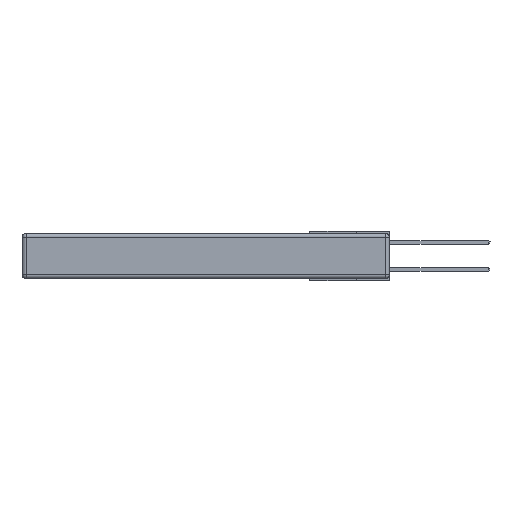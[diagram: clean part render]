
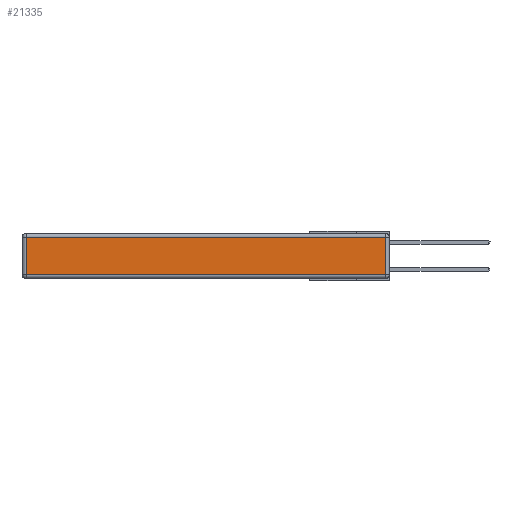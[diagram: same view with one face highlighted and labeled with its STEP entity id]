
A CAD part, left-side view. The second image highlights one B-rep face of the part: STEP entity #21335.
In plain terms, the highlighted planar face has unit normal (-1, 0, 0).
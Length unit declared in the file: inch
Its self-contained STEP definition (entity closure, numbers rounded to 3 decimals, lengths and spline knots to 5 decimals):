
#767 = CARTESIAN_POINT ( 'NONE',  ( 0., 0.03, -0.343 ) ) ;
#1240 = PLANE ( 'NONE',  #9766 ) ;
#1264 = DIRECTION ( 'NONE',  ( 0., 0., -1. ) ) ;
#2374 = CARTESIAN_POINT ( 'NONE',  ( 0., 0.03, -0.03 ) ) ;
#3075 = ORIENTED_EDGE ( 'NONE', *, *, #14206, .T. ) ;
#4648 = ORIENTED_EDGE ( 'NONE', *, *, #5697, .T. ) ;
#4725 = LINE ( 'NONE', #767, #12222 ) ;
#4911 = VECTOR ( 'NONE', #1264, 39.37008 ) ;
#5486 = CARTESIAN_POINT ( 'NONE',  ( 0., 0., -0.313 ) ) ;
#5515 = EDGE_CURVE ( 'NONE', #13794, #26208, #24156, .T. ) ;
#5697 = EDGE_CURVE ( 'NONE', #26208, #15934, #6198, .T. ) ;
#6198 = LINE ( 'NONE', #17628, #4911 ) ;
#6854 = VECTOR ( 'NONE', #22027, 39.37008 ) ;
#7051 = DIRECTION ( 'NONE',  ( 0., 0., 1. ) ) ;
#7062 = ORIENTED_EDGE ( 'NONE', *, *, #5515, .T. ) ;
#7544 = CARTESIAN_POINT ( 'NONE',  ( 0., 0.03, -0.313 ) ) ;
#8443 = CARTESIAN_POINT ( 'NONE',  ( 0., 2.72, -0.313 ) ) ;
#9766 = AXIS2_PLACEMENT_3D ( 'NONE', #26366, #11594, #20050 ) ;
#9810 = DIRECTION ( 'NONE',  ( 0., -1., 0. ) ) ;
#11027 = VECTOR ( 'NONE', #9810, 39.37008 ) ;
#11594 = DIRECTION ( 'NONE',  ( -1., 0., 0. ) ) ;
#12222 = VECTOR ( 'NONE', #7051, 39.37008 ) ;
#12968 = LINE ( 'NONE', #5486, #11027 ) ;
#13332 = VERTEX_POINT ( 'NONE', #7544 ) ;
#13659 = CARTESIAN_POINT ( 'NONE',  ( 0., 2.72, -0.03 ) ) ;
#13794 = VERTEX_POINT ( 'NONE', #2374 ) ;
#14050 = EDGE_LOOP ( 'NONE', ( #17841, #3075, #7062, #4648 ) ) ;
#14206 = EDGE_CURVE ( 'NONE', #13332, #13794, #4725, .T. ) ;
#15934 = VERTEX_POINT ( 'NONE', #8443 ) ;
#16028 = CARTESIAN_POINT ( 'NONE',  ( 0., 2.75, -0.03 ) ) ;
#17628 = CARTESIAN_POINT ( 'NONE',  ( 0., 2.72, -0.343 ) ) ;
#17841 = ORIENTED_EDGE ( 'NONE', *, *, #23421, .T. ) ;
#20050 = DIRECTION ( 'NONE',  ( 0., 0., 1. ) ) ;
#21335 = ADVANCED_FACE ( 'NONE', ( #22556 ), #1240, .T. ) ;
#22027 = DIRECTION ( 'NONE',  ( 0., 1., 0. ) ) ;
#22556 = FACE_OUTER_BOUND ( 'NONE', #14050, .T. ) ;
#23421 = EDGE_CURVE ( 'NONE', #15934, #13332, #12968, .T. ) ;
#24156 = LINE ( 'NONE', #16028, #6854 ) ;
#26208 = VERTEX_POINT ( 'NONE', #13659 ) ;
#26366 = CARTESIAN_POINT ( 'NONE',  ( 0., 0., -0.343 ) ) ;
